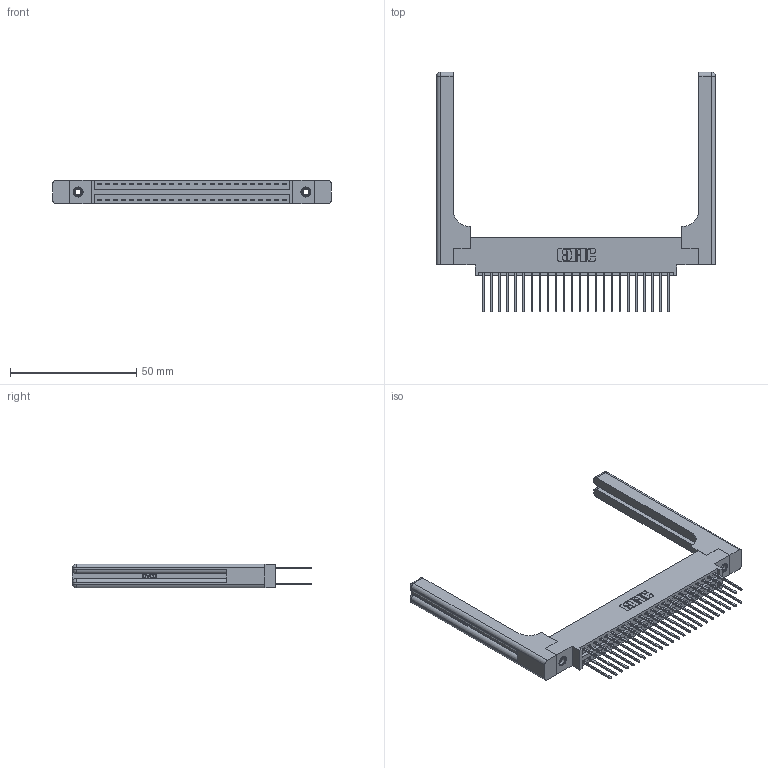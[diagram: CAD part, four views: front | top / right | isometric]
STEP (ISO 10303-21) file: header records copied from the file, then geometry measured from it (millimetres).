
FILE_DESCRIPTION (( 'STEP AP203' ), '1' );
FILE_NAME ('396-048-540-858.STEP', '2019-11-02T07:02:25', ( '' ), ( '' ), 'SwSTEP 2.0', 'SolidWorks 2016', '' );
FILE_SCHEMA (( 'CONFIG_CONTROL_DESIGN' ));
Length unit declared in the file: inch
Products named in the file (5): 346 Part_0.170 Offset - 0.156 Dia-TH; 345-292-001_345-293-140; 345-250-001_345-250-001-102; 346-220-058_345-220-058; 396-048-540-858
Assembly tree (53 placements, depth 2):
  396-048-540-858
    346 Part_0.170 Offset - 0.156 Dia-TH
    345-292-001_345-293-140  x48
    345-250-001_345-250-001-102  x2
    346-220-058_345-220-058  x2
Bounding box: 110.26 x 94.74 x 9.4 mm (x, y, z)
Volume: 18133.7 mm3; surface area: 20354.8 mm2
Topology: 53 solids, 53 shells, 2878 faces, 8447 edges, 5546 vertices
Faces by surface type: plane 1908, cylinder 910, bspline 36, cone 12, sphere 8, torus 4
Entity records: 23418 total; most frequent: CARTESIAN_POINT 4893, ORIENTED_EDGE 3624, DIRECTION 3296, EDGE_CURVE 1812, LINE 1492, VECTOR 1492, VERTEX_POINT 1198, AXIS2_PLACEMENT_3D 902
